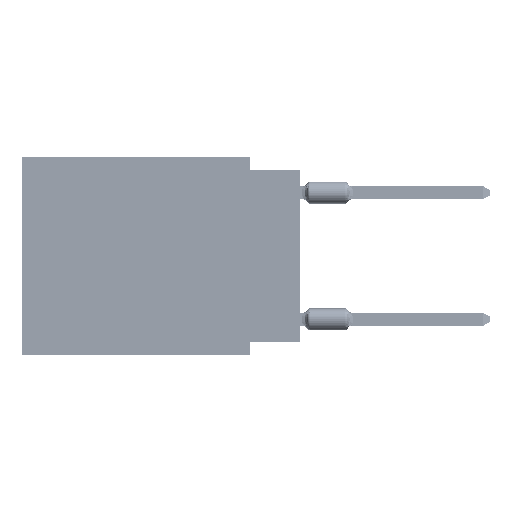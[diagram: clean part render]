
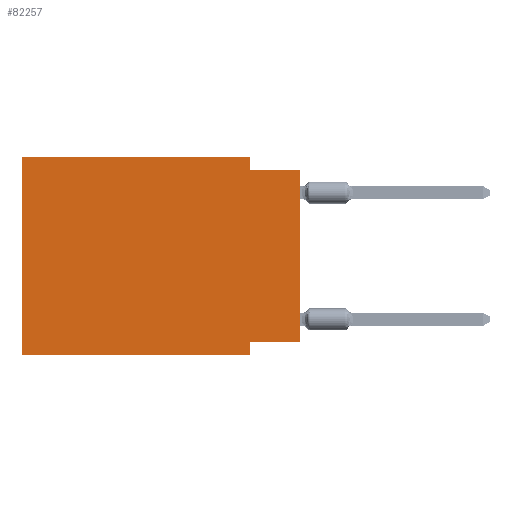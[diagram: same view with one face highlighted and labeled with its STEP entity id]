
A CAD part, left-side view. The second image highlights one B-rep face of the part: STEP entity #82257.
In plain terms, the highlighted planar face has unit normal (-1, 0, 0).
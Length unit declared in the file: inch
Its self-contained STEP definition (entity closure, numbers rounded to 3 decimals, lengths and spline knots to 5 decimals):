
#2341 = CARTESIAN_POINT ( 'NONE',  ( 0., 0.1, -0.365 ) ) ;
#4236 = FACE_OUTER_BOUND ( 'NONE', #21969, .T. ) ;
#5077 = CARTESIAN_POINT ( 'NONE',  ( 0., 0.1, -0.39 ) ) ;
#9617 = VERTEX_POINT ( 'NONE', #32981 ) ;
#10538 = ORIENTED_EDGE ( 'NONE', *, *, #12585, .T. ) ;
#12585 = EDGE_CURVE ( 'NONE', #9617, #24169, #48473, .T. ) ;
#12931 = EDGE_CURVE ( 'NONE', #25773, #79410, #53692, .T. ) ;
#13050 = ORIENTED_EDGE ( 'NONE', *, *, #85723, .F. ) ;
#15986 = VECTOR ( 'NONE', #19252, 39.37008 ) ;
#19252 = DIRECTION ( 'NONE',  ( 0., -1., 0. ) ) ;
#20111 = CARTESIAN_POINT ( 'NONE',  ( 0., 0.55, 0. ) ) ;
#20136 = DIRECTION ( 'NONE',  ( 0., 1., 0. ) ) ;
#20869 = VECTOR ( 'NONE', #20136, 39.37008 ) ;
#21969 = EDGE_LOOP ( 'NONE', ( #33743, #65597, #65779, #53230, #77715, #10538, #76200, #13050 ) ) ;
#24108 = CARTESIAN_POINT ( 'NONE',  ( 0., 0.55, 0. ) ) ;
#24169 = VERTEX_POINT ( 'NONE', #57401 ) ;
#25174 = EDGE_CURVE ( 'NONE', #9617, #25773, #40271, .T. ) ;
#25360 = CARTESIAN_POINT ( 'NONE',  ( 0., 0., 0. ) ) ;
#25773 = VERTEX_POINT ( 'NONE', #78954 ) ;
#25898 = EDGE_CURVE ( 'NONE', #57055, #74506, #52422, .T. ) ;
#26401 = VECTOR ( 'NONE', #68716, 39.37008 ) ;
#28602 = VECTOR ( 'NONE', #55965, 39.37008 ) ;
#29361 = EDGE_CURVE ( 'NONE', #38396, #74506, #64671, .T. ) ;
#30811 = CARTESIAN_POINT ( 'NONE',  ( 0., 0., -0.025 ) ) ;
#32981 = CARTESIAN_POINT ( 'NONE',  ( 0., 0.55, -0.39 ) ) ;
#33524 = EDGE_CURVE ( 'NONE', #79410, #57055, #66963, .T. ) ;
#33743 = ORIENTED_EDGE ( 'NONE', *, *, #29361, .T. ) ;
#33846 = CARTESIAN_POINT ( 'NONE',  ( 0., 0., -0.365 ) ) ;
#38331 = DIRECTION ( 'NONE',  ( 0., -1., 0. ) ) ;
#38396 = VERTEX_POINT ( 'NONE', #59416 ) ;
#40271 = LINE ( 'NONE', #40701, #56625 ) ;
#40701 = CARTESIAN_POINT ( 'NONE',  ( 0., 0.55, 0. ) ) ;
#45285 = DIRECTION ( 'NONE',  ( 1., 0., 0. ) ) ;
#48473 = LINE ( 'NONE', #49770, #28602 ) ;
#49770 = CARTESIAN_POINT ( 'NONE',  ( 0., 0.55, -0.39 ) ) ;
#50612 = PLANE ( 'NONE',  #85488 ) ;
#50919 = CARTESIAN_POINT ( 'NONE',  ( 0., 0.1, -0.025 ) ) ;
#51906 = DIRECTION ( 'NONE',  ( 0., 0., -1. ) ) ;
#52422 = LINE ( 'NONE', #30811, #80896 ) ;
#53230 = ORIENTED_EDGE ( 'NONE', *, *, #12931, .F. ) ;
#53692 = LINE ( 'NONE', #20111, #15986 ) ;
#54593 = CARTESIAN_POINT ( 'NONE',  ( 0., 0.1, 0. ) ) ;
#55965 = DIRECTION ( 'NONE',  ( 0., -1., 0. ) ) ;
#56625 = VECTOR ( 'NONE', #61440, 39.37008 ) ;
#57055 = VERTEX_POINT ( 'NONE', #50919 ) ;
#57401 = CARTESIAN_POINT ( 'NONE',  ( 0., 0.1, -0.39 ) ) ;
#58559 = VECTOR ( 'NONE', #85439, 39.37008 ) ;
#59416 = CARTESIAN_POINT ( 'NONE',  ( 0., 0., -0.365 ) ) ;
#61440 = DIRECTION ( 'NONE',  ( 0., 0., 1. ) ) ;
#64671 = LINE ( 'NONE', #25360, #58559 ) ;
#65597 = ORIENTED_EDGE ( 'NONE', *, *, #25898, .F. ) ;
#65779 = ORIENTED_EDGE ( 'NONE', *, *, #33524, .F. ) ;
#66963 = LINE ( 'NONE', #54593, #26401 ) ;
#68716 = DIRECTION ( 'NONE',  ( 0., 0., -1. ) ) ;
#70380 = VECTOR ( 'NONE', #70895, 39.37008 ) ;
#70464 = LINE ( 'NONE', #5077, #70380 ) ;
#70895 = DIRECTION ( 'NONE',  ( 0., 0., -1. ) ) ;
#72118 = CARTESIAN_POINT ( 'NONE',  ( 0., 0., -0.025 ) ) ;
#73296 = CARTESIAN_POINT ( 'NONE',  ( 0., 0.1, 0. ) ) ;
#73603 = LINE ( 'NONE', #33846, #20869 ) ;
#74506 = VERTEX_POINT ( 'NONE', #72118 ) ;
#76200 = ORIENTED_EDGE ( 'NONE', *, *, #87254, .F. ) ;
#77715 = ORIENTED_EDGE ( 'NONE', *, *, #25174, .F. ) ;
#78954 = CARTESIAN_POINT ( 'NONE',  ( 0., 0.55, 0. ) ) ;
#79410 = VERTEX_POINT ( 'NONE', #73296 ) ;
#80896 = VECTOR ( 'NONE', #38331, 39.37008 ) ;
#82257 = ADVANCED_FACE ( 'NONE', ( #4236 ), #50612, .F. ) ;
#85439 = DIRECTION ( 'NONE',  ( 0., 0., 1. ) ) ;
#85488 = AXIS2_PLACEMENT_3D ( 'NONE', #24108, #45285, #51906 ) ;
#85723 = EDGE_CURVE ( 'NONE', #38396, #86342, #73603, .T. ) ;
#86342 = VERTEX_POINT ( 'NONE', #2341 ) ;
#87254 = EDGE_CURVE ( 'NONE', #86342, #24169, #70464, .T. ) ;
